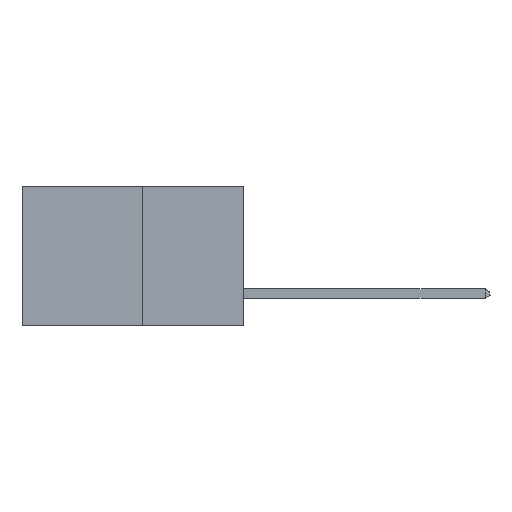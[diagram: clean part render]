
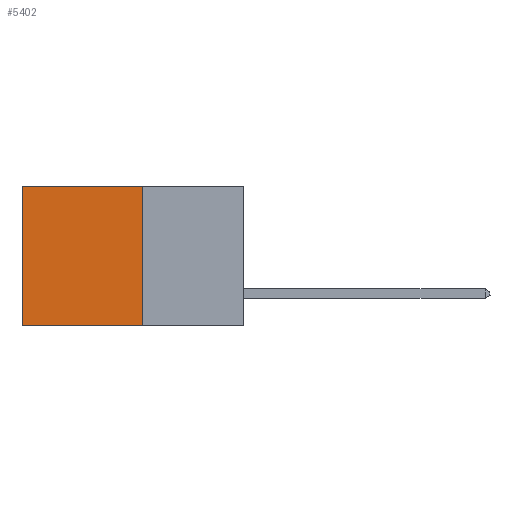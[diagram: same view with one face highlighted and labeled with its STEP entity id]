
A CAD part, left-side view. The second image highlights one B-rep face of the part: STEP entity #5402.
In plain terms, the highlighted planar face has unit normal (-1, 0, 0).
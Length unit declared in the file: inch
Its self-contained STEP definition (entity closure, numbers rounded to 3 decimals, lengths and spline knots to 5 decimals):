
#95 = EDGE_CURVE ( 'NONE', #3341, #11206, #663, .T. ) ;
#663 = LINE ( 'NONE', #8733, #9431 ) ;
#739 = VERTEX_POINT ( 'NONE', #3768 ) ;
#935 = DIRECTION ( 'NONE',  ( 0., 1., 0. ) ) ;
#1226 = DIRECTION ( 'NONE',  ( 0., 0., -1. ) ) ;
#1272 = DIRECTION ( 'NONE',  ( 1., 0., 0. ) ) ;
#1320 = PLANE ( 'NONE',  #6515 ) ;
#1344 = CARTESIAN_POINT ( 'NONE',  ( 0.277, 0.27, -0.37 ) ) ;
#2813 = VECTOR ( 'NONE', #13604, 39.37008 ) ;
#3341 = VERTEX_POINT ( 'NONE', #13281 ) ;
#3768 = CARTESIAN_POINT ( 'NONE',  ( 0.277, 0.27, -0.37 ) ) ;
#4365 = DIRECTION ( 'NONE',  ( 0., 0., -1. ) ) ;
#5402 = ADVANCED_FACE ( 'NONE', ( #9885 ), #1320, .F. ) ;
#6515 = AXIS2_PLACEMENT_3D ( 'NONE', #1344, #1272, #1226 ) ;
#7236 = LINE ( 'NONE', #8734, #2813 ) ;
#8194 = ORIENTED_EDGE ( 'NONE', *, *, #14403, .F. ) ;
#8733 = CARTESIAN_POINT ( 'NONE',  ( 0.277, 0.27, 0. ) ) ;
#8734 = CARTESIAN_POINT ( 'NONE',  ( 0.277, 0.27, -0.37 ) ) ;
#9431 = VECTOR ( 'NONE', #13933, 39.37008 ) ;
#9727 = VECTOR ( 'NONE', #4365, 39.37008 ) ;
#9745 = ORIENTED_EDGE ( 'NONE', *, *, #95, .T. ) ;
#9885 = FACE_OUTER_BOUND ( 'NONE', #19829, .T. ) ;
#11206 = VERTEX_POINT ( 'NONE', #14310 ) ;
#11528 = VERTEX_POINT ( 'NONE', #16640 ) ;
#11582 = EDGE_CURVE ( 'NONE', #3341, #739, #7236, .T. ) ;
#12537 = CARTESIAN_POINT ( 'NONE',  ( 0.277, 0.59, -0.37 ) ) ;
#13147 = EDGE_CURVE ( 'NONE', #11206, #11528, #15001, .T. ) ;
#13281 = CARTESIAN_POINT ( 'NONE',  ( 0.277, 0.27, 0. ) ) ;
#13604 = DIRECTION ( 'NONE',  ( 0., 0., -1. ) ) ;
#13933 = DIRECTION ( 'NONE',  ( 0., 1., 0. ) ) ;
#14310 = CARTESIAN_POINT ( 'NONE',  ( 0.277, 0.59, 0. ) ) ;
#14403 = EDGE_CURVE ( 'NONE', #739, #11528, #18706, .T. ) ;
#14444 = VECTOR ( 'NONE', #935, 39.37008 ) ;
#15001 = LINE ( 'NONE', #12537, #9727 ) ;
#15545 = CARTESIAN_POINT ( 'NONE',  ( 0.277, 0.27, -0.37 ) ) ;
#16640 = CARTESIAN_POINT ( 'NONE',  ( 0.277, 0.59, -0.37 ) ) ;
#18706 = LINE ( 'NONE', #15545, #14444 ) ;
#18959 = ORIENTED_EDGE ( 'NONE', *, *, #11582, .F. ) ;
#19829 = EDGE_LOOP ( 'NONE', ( #20492, #8194, #18959, #9745 ) ) ;
#20492 = ORIENTED_EDGE ( 'NONE', *, *, #13147, .T. ) ;
